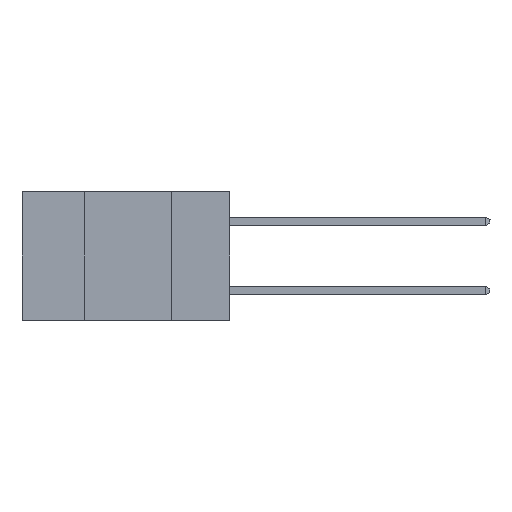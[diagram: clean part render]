
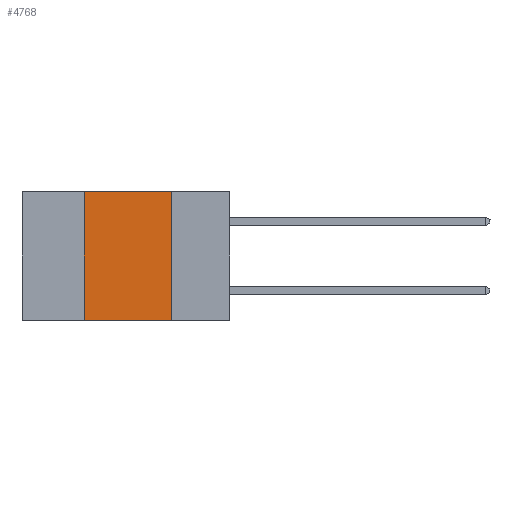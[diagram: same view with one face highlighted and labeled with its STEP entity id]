
A CAD part, left-side view. The second image highlights one B-rep face of the part: STEP entity #4768.
In plain terms, the highlighted planar face has unit normal (-1, 0, 0).
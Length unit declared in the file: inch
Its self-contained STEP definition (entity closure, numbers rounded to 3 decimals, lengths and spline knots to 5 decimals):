
#455 = VERTEX_POINT ( 'NONE', #685 ) ;
#685 = CARTESIAN_POINT ( 'NONE',  ( 0., 0.17, -0.37 ) ) ;
#1171 = EDGE_CURVE ( 'NONE', #7139, #455, #5925, .T. ) ;
#1290 = CARTESIAN_POINT ( 'NONE',  ( 0., 0.6, 0. ) ) ;
#1990 = VECTOR ( 'NONE', #6978, 39.37008 ) ;
#2712 = CARTESIAN_POINT ( 'NONE',  ( 0., 0.6, 0. ) ) ;
#4130 = EDGE_CURVE ( 'NONE', #11438, #455, #13801, .T. ) ;
#4768 = ADVANCED_FACE ( 'NONE', ( #10125 ), #13236, .F. ) ;
#4770 = EDGE_LOOP ( 'NONE', ( #11775, #10592, #4822, #5138 ) ) ;
#4822 = ORIENTED_EDGE ( 'NONE', *, *, #4966, .F. ) ;
#4878 = DIRECTION ( 'NONE',  ( 0., 0., -1. ) ) ;
#4966 = EDGE_CURVE ( 'NONE', #7139, #8279, #8154, .T. ) ;
#5138 = ORIENTED_EDGE ( 'NONE', *, *, #1171, .T. ) ;
#5187 = DIRECTION ( 'NONE',  ( 0., 0., -1. ) ) ;
#5418 = LINE ( 'NONE', #1290, #8949 ) ;
#5925 = LINE ( 'NONE', #9066, #1990 ) ;
#5971 = AXIS2_PLACEMENT_3D ( 'NONE', #2712, #10259, #4878 ) ;
#6978 = DIRECTION ( 'NONE',  ( 0., -1., 0. ) ) ;
#7139 = VERTEX_POINT ( 'NONE', #12060 ) ;
#8154 = LINE ( 'NONE', #10340, #12702 ) ;
#8279 = VERTEX_POINT ( 'NONE', #11989 ) ;
#8617 = DIRECTION ( 'NONE',  ( 0., 0., 1. ) ) ;
#8949 = VECTOR ( 'NONE', #9949, 39.37008 ) ;
#9066 = CARTESIAN_POINT ( 'NONE',  ( 0., 0.6, -0.37 ) ) ;
#9912 = EDGE_CURVE ( 'NONE', #8279, #11438, #5418, .T. ) ;
#9949 = DIRECTION ( 'NONE',  ( 0., -1., 0. ) ) ;
#10125 = FACE_OUTER_BOUND ( 'NONE', #4770, .T. ) ;
#10228 = CARTESIAN_POINT ( 'NONE',  ( 0., 0.17, 0. ) ) ;
#10259 = DIRECTION ( 'NONE',  ( 1., 0., 0. ) ) ;
#10340 = CARTESIAN_POINT ( 'NONE',  ( 0., 0.42, -0.37 ) ) ;
#10592 = ORIENTED_EDGE ( 'NONE', *, *, #9912, .F. ) ;
#10639 = CARTESIAN_POINT ( 'NONE',  ( 0., 0.17, -0.37 ) ) ;
#11438 = VERTEX_POINT ( 'NONE', #10228 ) ;
#11775 = ORIENTED_EDGE ( 'NONE', *, *, #4130, .F. ) ;
#11989 = CARTESIAN_POINT ( 'NONE',  ( 0., 0.42, 0. ) ) ;
#12060 = CARTESIAN_POINT ( 'NONE',  ( 0., 0.42, -0.37 ) ) ;
#12702 = VECTOR ( 'NONE', #8617, 39.37008 ) ;
#13236 = PLANE ( 'NONE',  #5971 ) ;
#13801 = LINE ( 'NONE', #10639, #13811 ) ;
#13811 = VECTOR ( 'NONE', #5187, 39.37008 ) ;
